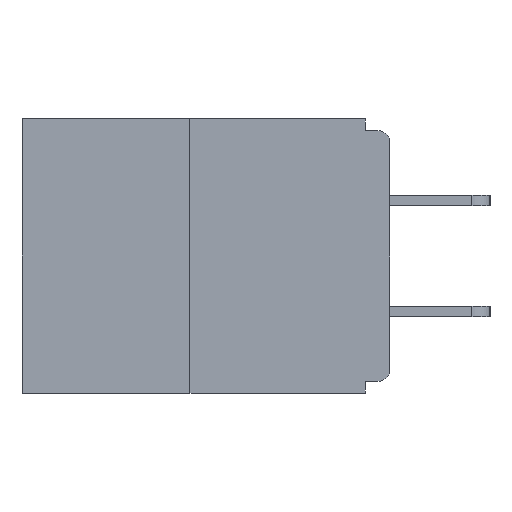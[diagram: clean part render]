
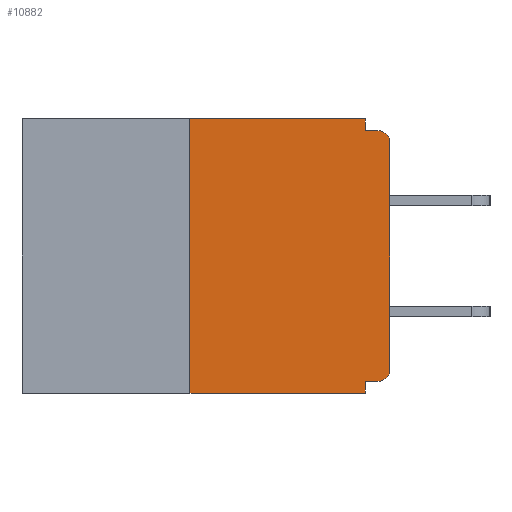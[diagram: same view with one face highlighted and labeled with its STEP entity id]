
A CAD part, left-side view. The second image highlights one B-rep face of the part: STEP entity #10882.
In plain terms, the highlighted planar face has unit normal (-1, 0, 0).
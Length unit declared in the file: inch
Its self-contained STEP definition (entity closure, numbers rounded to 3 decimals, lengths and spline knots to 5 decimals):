
#502 = DIRECTION ( 'NONE',  ( 0., 0., -1. ) ) ;
#565 = VERTEX_POINT ( 'NONE', #14677 ) ;
#627 = EDGE_CURVE ( 'NONE', #6764, #565, #11957, .T. ) ;
#1120 = LINE ( 'NONE', #6032, #9262 ) ;
#1506 = CARTESIAN_POINT ( 'NONE',  ( 0., 0.031, 0. ) ) ;
#1715 = CARTESIAN_POINT ( 'NONE',  ( 0., 0.031, -0.328 ) ) ;
#1770 = CIRCLE ( 'NONE', #14437, 0.015 ) ;
#1789 = EDGE_CURVE ( 'NONE', #13228, #3120, #7232, .T. ) ;
#1826 = EDGE_CURVE ( 'NONE', #4805, #12283, #9570, .T. ) ;
#2313 = ORIENTED_EDGE ( 'NONE', *, *, #627, .T. ) ;
#2411 = EDGE_CURVE ( 'NONE', #13228, #12283, #9067, .T. ) ;
#2722 = DIRECTION ( 'NONE',  ( 1., 0., 0. ) ) ;
#3120 = VERTEX_POINT ( 'NONE', #14556 ) ;
#3277 = DIRECTION ( 'NONE',  ( 0., -1., 0. ) ) ;
#3766 = VERTEX_POINT ( 'NONE', #6552 ) ;
#3876 = DIRECTION ( 'NONE',  ( 0., 0., -1. ) ) ;
#3943 = ORIENTED_EDGE ( 'NONE', *, *, #1826, .F. ) ;
#4198 = EDGE_CURVE ( 'NONE', #6764, #4805, #1120, .T. ) ;
#4239 = ORIENTED_EDGE ( 'NONE', *, *, #5900, .T. ) ;
#4273 = ORIENTED_EDGE ( 'NONE', *, *, #4198, .F. ) ;
#4275 = VERTEX_POINT ( 'NONE', #10240 ) ;
#4302 = DIRECTION ( 'NONE',  ( 0., 0., -1. ) ) ;
#4805 = VERTEX_POINT ( 'NONE', #1715 ) ;
#5191 = VERTEX_POINT ( 'NONE', #13108 ) ;
#5276 = EDGE_CURVE ( 'NONE', #3120, #9904, #10823, .T. ) ;
#5432 = DIRECTION ( 'NONE',  ( 0., 1., 0. ) ) ;
#5449 = EDGE_CURVE ( 'NONE', #5191, #3766, #7353, .T. ) ;
#5486 = PLANE ( 'NONE',  #11788 ) ;
#5832 = CARTESIAN_POINT ( 'NONE',  ( 0., 0.031, -0.343 ) ) ;
#5900 = EDGE_CURVE ( 'NONE', #4275, #3766, #1770, .T. ) ;
#6032 = CARTESIAN_POINT ( 'NONE',  ( 0., 0., -0.328 ) ) ;
#6417 = VECTOR ( 'NONE', #14354, 39.37008 ) ;
#6551 = DIRECTION ( 'NONE',  ( 0., -1., 0. ) ) ;
#6552 = CARTESIAN_POINT ( 'NONE',  ( 0., 0.015, -0.015 ) ) ;
#6764 = VERTEX_POINT ( 'NONE', #14706 ) ;
#6891 = CARTESIAN_POINT ( 'NONE',  ( 0., 0.25, -0.343 ) ) ;
#7023 = ORIENTED_EDGE ( 'NONE', *, *, #5276, .F. ) ;
#7232 = LINE ( 'NONE', #9402, #6417 ) ;
#7353 = LINE ( 'NONE', #7895, #8407 ) ;
#7509 = EDGE_LOOP ( 'NONE', ( #7023, #8177, #14743, #3943, #4273, #2313, #8459, #4239, #15074, #15311 ) ) ;
#7860 = CARTESIAN_POINT ( 'NONE',  ( 0., 0.015, -0.313 ) ) ;
#7895 = CARTESIAN_POINT ( 'NONE',  ( 0., 0., -0.015 ) ) ;
#8177 = ORIENTED_EDGE ( 'NONE', *, *, #1789, .F. ) ;
#8407 = VECTOR ( 'NONE', #12597, 39.37008 ) ;
#8459 = ORIENTED_EDGE ( 'NONE', *, *, #10541, .T. ) ;
#8517 = AXIS2_PLACEMENT_3D ( 'NONE', #7860, #12556, #3876 ) ;
#9067 = LINE ( 'NONE', #13693, #15153 ) ;
#9262 = VECTOR ( 'NONE', #5432, 39.37008 ) ;
#9402 = CARTESIAN_POINT ( 'NONE',  ( 0., 0.25, 0. ) ) ;
#9525 = VECTOR ( 'NONE', #4302, 39.37008 ) ;
#9570 = LINE ( 'NONE', #5832, #11326 ) ;
#9904 = VERTEX_POINT ( 'NONE', #1506 ) ;
#10123 = FACE_OUTER_BOUND ( 'NONE', #7509, .T. ) ;
#10240 = CARTESIAN_POINT ( 'NONE',  ( 0., 0., -0.03 ) ) ;
#10452 = CARTESIAN_POINT ( 'NONE',  ( 0., 0., 0. ) ) ;
#10541 = EDGE_CURVE ( 'NONE', #565, #4275, #12885, .T. ) ;
#10784 = DIRECTION ( 'NONE',  ( 0., 0., -1. ) ) ;
#10823 = LINE ( 'NONE', #14568, #14613 ) ;
#10882 = ADVANCED_FACE ( 'NONE', ( #10123 ), #5486, .F. ) ;
#11326 = VECTOR ( 'NONE', #10784, 39.37008 ) ;
#11414 = CARTESIAN_POINT ( 'NONE',  ( 0., 0.46, 0. ) ) ;
#11443 = CARTESIAN_POINT ( 'NONE',  ( 0., 0.015, -0.03 ) ) ;
#11703 = LINE ( 'NONE', #12753, #9525 ) ;
#11788 = AXIS2_PLACEMENT_3D ( 'NONE', #11414, #2722, #502 ) ;
#11957 = CIRCLE ( 'NONE', #8517, 0.015 ) ;
#12283 = VERTEX_POINT ( 'NONE', #13095 ) ;
#12556 = DIRECTION ( 'NONE',  ( -1., 0., 0. ) ) ;
#12597 = DIRECTION ( 'NONE',  ( 0., -1., 0. ) ) ;
#12667 = DIRECTION ( 'NONE',  ( -1., 0., 0. ) ) ;
#12753 = CARTESIAN_POINT ( 'NONE',  ( 0., 0.031, 0. ) ) ;
#12885 = LINE ( 'NONE', #10452, #13164 ) ;
#13095 = CARTESIAN_POINT ( 'NONE',  ( 0., 0.031, -0.343 ) ) ;
#13108 = CARTESIAN_POINT ( 'NONE',  ( 0., 0.031, -0.015 ) ) ;
#13164 = VECTOR ( 'NONE', #15403, 39.37008 ) ;
#13228 = VERTEX_POINT ( 'NONE', #6891 ) ;
#13693 = CARTESIAN_POINT ( 'NONE',  ( 0., 0.46, -0.343 ) ) ;
#13843 = EDGE_CURVE ( 'NONE', #9904, #5191, #11703, .T. ) ;
#13879 = DIRECTION ( 'NONE',  ( 0., 0., -1. ) ) ;
#14354 = DIRECTION ( 'NONE',  ( 0., 0., 1. ) ) ;
#14437 = AXIS2_PLACEMENT_3D ( 'NONE', #11443, #12667, #13879 ) ;
#14556 = CARTESIAN_POINT ( 'NONE',  ( 0., 0.25, 0. ) ) ;
#14568 = CARTESIAN_POINT ( 'NONE',  ( 0., 0.46, 0. ) ) ;
#14613 = VECTOR ( 'NONE', #3277, 39.37008 ) ;
#14677 = CARTESIAN_POINT ( 'NONE',  ( 0., 0., -0.313 ) ) ;
#14706 = CARTESIAN_POINT ( 'NONE',  ( 0., 0.015, -0.328 ) ) ;
#14743 = ORIENTED_EDGE ( 'NONE', *, *, #2411, .T. ) ;
#15074 = ORIENTED_EDGE ( 'NONE', *, *, #5449, .F. ) ;
#15153 = VECTOR ( 'NONE', #6551, 39.37008 ) ;
#15311 = ORIENTED_EDGE ( 'NONE', *, *, #13843, .F. ) ;
#15403 = DIRECTION ( 'NONE',  ( 0., 0., 1. ) ) ;
